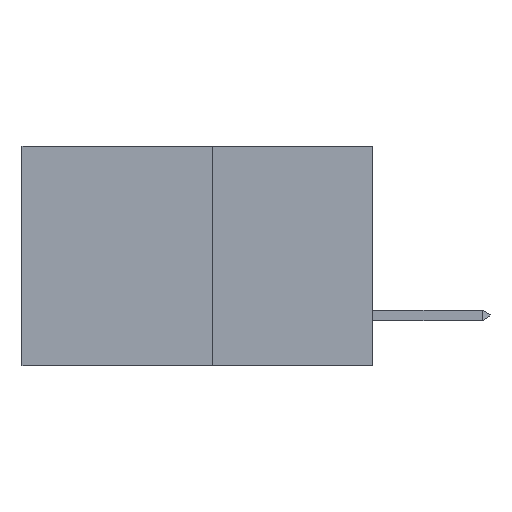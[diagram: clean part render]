
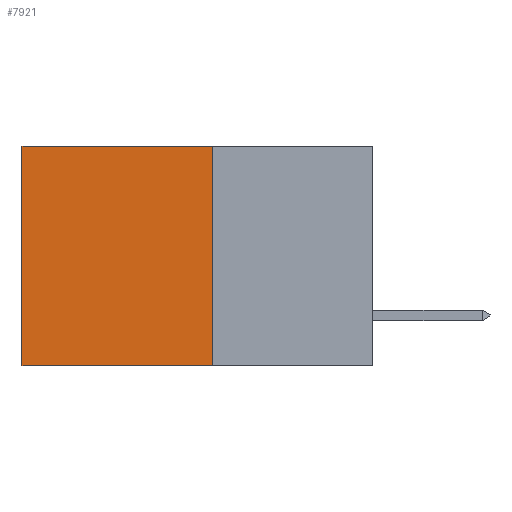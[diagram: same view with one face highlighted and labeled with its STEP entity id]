
A CAD part, left-side view. The second image highlights one B-rep face of the part: STEP entity #7921.
In plain terms, the highlighted planar face has unit normal (-1, 0, 0).
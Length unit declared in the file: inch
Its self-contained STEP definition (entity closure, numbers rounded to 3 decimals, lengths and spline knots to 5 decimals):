
#226 = LINE ( 'NONE', #5422, #3180 ) ;
#249 = VECTOR ( 'NONE', #6843, 39.37008 ) ;
#324 = ORIENTED_EDGE ( 'NONE', *, *, #10857, .F. ) ;
#332 = EDGE_CURVE ( 'NONE', #7724, #8181, #8840, .T. ) ;
#471 = VERTEX_POINT ( 'NONE', #10361 ) ;
#703 = ORIENTED_EDGE ( 'NONE', *, *, #5824, .F. ) ;
#752 = AXIS2_PLACEMENT_3D ( 'NONE', #2421, #8815, #3340 ) ;
#1221 = CARTESIAN_POINT ( 'NONE',  ( 0.277, 0.27, -0.37 ) ) ;
#1432 = LINE ( 'NONE', #2847, #8252 ) ;
#2421 = CARTESIAN_POINT ( 'NONE',  ( 0.277, 0.27, -0.37 ) ) ;
#2847 = CARTESIAN_POINT ( 'NONE',  ( 0.277, 0.27, -0.37 ) ) ;
#3180 = VECTOR ( 'NONE', #6392, 39.37008 ) ;
#3299 = PLANE ( 'NONE',  #752 ) ;
#3340 = DIRECTION ( 'NONE',  ( 0., 0., -1. ) ) ;
#4264 = VECTOR ( 'NONE', #6879, 39.37008 ) ;
#5422 = CARTESIAN_POINT ( 'NONE',  ( 0.277, 0.27, 0. ) ) ;
#5629 = VERTEX_POINT ( 'NONE', #9818 ) ;
#5738 = ORIENTED_EDGE ( 'NONE', *, *, #332, .T. ) ;
#5824 = EDGE_CURVE ( 'NONE', #5629, #471, #1432, .T. ) ;
#6050 = ORIENTED_EDGE ( 'NONE', *, *, #6619, .T. ) ;
#6392 = DIRECTION ( 'NONE',  ( 0., 1., 0. ) ) ;
#6619 = EDGE_CURVE ( 'NONE', #5629, #7724, #226, .T. ) ;
#6843 = DIRECTION ( 'NONE',  ( 0., 1., 0. ) ) ;
#6879 = DIRECTION ( 'NONE',  ( 0., 0., -1. ) ) ;
#7724 = VERTEX_POINT ( 'NONE', #11212 ) ;
#7825 = LINE ( 'NONE', #1221, #249 ) ;
#7921 = ADVANCED_FACE ( 'NONE', ( #9550 ), #3299, .F. ) ;
#8181 = VERTEX_POINT ( 'NONE', #9072 ) ;
#8252 = VECTOR ( 'NONE', #8370, 39.37008 ) ;
#8370 = DIRECTION ( 'NONE',  ( 0., 0., -1. ) ) ;
#8815 = DIRECTION ( 'NONE',  ( 1., 0., 0. ) ) ;
#8840 = LINE ( 'NONE', #9946, #4264 ) ;
#9072 = CARTESIAN_POINT ( 'NONE',  ( 0.277, 0.59, -0.37 ) ) ;
#9550 = FACE_OUTER_BOUND ( 'NONE', #11591, .T. ) ;
#9818 = CARTESIAN_POINT ( 'NONE',  ( 0.277, 0.27, 0. ) ) ;
#9946 = CARTESIAN_POINT ( 'NONE',  ( 0.277, 0.59, -0.37 ) ) ;
#10361 = CARTESIAN_POINT ( 'NONE',  ( 0.277, 0.27, -0.37 ) ) ;
#10857 = EDGE_CURVE ( 'NONE', #471, #8181, #7825, .T. ) ;
#11212 = CARTESIAN_POINT ( 'NONE',  ( 0.277, 0.59, 0. ) ) ;
#11591 = EDGE_LOOP ( 'NONE', ( #5738, #324, #703, #6050 ) ) ;
